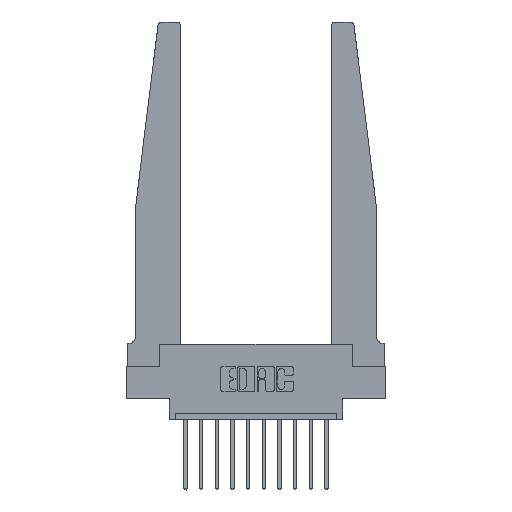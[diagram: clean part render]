
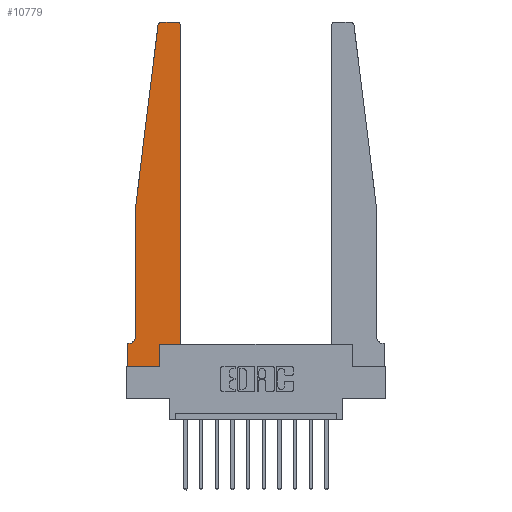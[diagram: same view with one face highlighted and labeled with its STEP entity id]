
A CAD part, top view. The second image highlights one B-rep face of the part: STEP entity #10779.
In plain terms, the highlighted planar face has unit normal (0, 0, 1).
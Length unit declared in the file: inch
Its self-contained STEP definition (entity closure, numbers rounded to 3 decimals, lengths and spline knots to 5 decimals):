
#94 = EDGE_CURVE ( 'NONE', #14381, #6517, #8369, .T. ) ;
#203 = ORIENTED_EDGE ( 'NONE', *, *, #13547, .T. ) ;
#266 = EDGE_CURVE ( 'NONE', #2479, #7509, #4620, .T. ) ;
#385 = DIRECTION ( 'NONE',  ( -1., 0., 0. ) ) ;
#574 = EDGE_CURVE ( 'NONE', #6517, #11387, #15032, .T. ) ;
#618 = CARTESIAN_POINT ( 'NONE',  ( 0.24675, 2.72367, 0.37 ) ) ;
#689 = EDGE_CURVE ( 'NONE', #11387, #13589, #2000, .T. ) ;
#945 = CARTESIAN_POINT ( 'NONE',  ( 0., 0., 0.37 ) ) ;
#994 = LINE ( 'NONE', #6696, #12910 ) ;
#1380 = DIRECTION ( 'NONE',  ( 0., 1., 0. ) ) ;
#1482 = VECTOR ( 'NONE', #5761, 39.37008 ) ;
#1669 = LINE ( 'NONE', #9377, #1482 ) ;
#1726 = CARTESIAN_POINT ( 'NONE',  ( 0., 0.1875, 0.37 ) ) ;
#1998 = ORIENTED_EDGE ( 'NONE', *, *, #94, .T. ) ;
#2000 = CIRCLE ( 'NONE', #4517, 0.05 ) ;
#2479 = VERTEX_POINT ( 'NONE', #14240 ) ;
#2509 = DIRECTION ( 'NONE',  ( 1., 0., 0. ) ) ;
#2697 = CARTESIAN_POINT ( 'NONE',  ( 0., 0.1875, 0.37 ) ) ;
#2718 = LINE ( 'NONE', #7629, #4381 ) ;
#2761 = EDGE_CURVE ( 'NONE', #13950, #14381, #3638, .T. ) ;
#2949 = ORIENTED_EDGE ( 'NONE', *, *, #2761, .T. ) ;
#3106 = ORIENTED_EDGE ( 'NONE', *, *, #574, .T. ) ;
#3379 = CARTESIAN_POINT ( 'NONE',  ( 0.2605, 0.18, 0.37 ) ) ;
#3638 = CIRCLE ( 'NONE', #13577, 0.03 ) ;
#3648 = CARTESIAN_POINT ( 'NONE',  ( 0.395, 2.75, 0.37 ) ) ;
#3850 = CARTESIAN_POINT ( 'NONE',  ( 0.27653, 2.72, 0.37 ) ) ;
#3911 = DIRECTION ( 'NONE',  ( 1., 0., 0. ) ) ;
#4058 = ORIENTED_EDGE ( 'NONE', *, *, #11117, .T. ) ;
#4083 = LINE ( 'NONE', #11923, #5564 ) ;
#4130 = CARTESIAN_POINT ( 'NONE',  ( 0.25, 2.75, 0.37 ) ) ;
#4381 = VECTOR ( 'NONE', #7582, 39.37008 ) ;
#4398 = CARTESIAN_POINT ( 'NONE',  ( 0.27653, 2.75, 0.37 ) ) ;
#4490 = CIRCLE ( 'NONE', #13267, 0.03 ) ;
#4517 = AXIS2_PLACEMENT_3D ( 'NONE', #7605, #12346, #385 ) ;
#4620 = LINE ( 'NONE', #8796, #14852 ) ;
#5473 = CARTESIAN_POINT ( 'NONE',  ( 0.065, 0.2375, 0.37 ) ) ;
#5564 = VECTOR ( 'NONE', #1380, 39.37008 ) ;
#5761 = DIRECTION ( 'NONE',  ( 0., -1., 0. ) ) ;
#5963 = CARTESIAN_POINT ( 'NONE',  ( 0.065, 1.25, 0.37 ) ) ;
#6069 = CARTESIAN_POINT ( 'NONE',  ( 0.065, 1.25, 0.37 ) ) ;
#6158 = ORIENTED_EDGE ( 'NONE', *, *, #15377, .T. ) ;
#6278 = VECTOR ( 'NONE', #8907, 39.37008 ) ;
#6314 = CARTESIAN_POINT ( 'NONE',  ( 0.015, 0.1875, 0.37 ) ) ;
#6318 = CARTESIAN_POINT ( 'NONE',  ( 0.065, 1.25, 0.37 ) ) ;
#6517 = VERTEX_POINT ( 'NONE', #5963 ) ;
#6696 = CARTESIAN_POINT ( 'NONE',  ( 0., 0., 0.37 ) ) ;
#7171 = CARTESIAN_POINT ( 'NONE',  ( 0.395, 2.72, 0.37 ) ) ;
#7348 = ORIENTED_EDGE ( 'NONE', *, *, #10474, .T. ) ;
#7509 = VERTEX_POINT ( 'NONE', #3379 ) ;
#7582 = DIRECTION ( 'NONE',  ( -1., 0., 0. ) ) ;
#7605 = CARTESIAN_POINT ( 'NONE',  ( 0.015, 0.2375, 0.37 ) ) ;
#7629 = CARTESIAN_POINT ( 'NONE',  ( 0.065, 0.1875, 0.37 ) ) ;
#7836 = VERTEX_POINT ( 'NONE', #8964 ) ;
#8135 = VECTOR ( 'NONE', #9257, 39.37008 ) ;
#8369 = LINE ( 'NONE', #6069, #10794 ) ;
#8403 = EDGE_CURVE ( 'NONE', #8819, #13950, #13340, .T. ) ;
#8549 = DIRECTION ( 'NONE',  ( 0., 0., 1. ) ) ;
#8582 = AXIS2_PLACEMENT_3D ( 'NONE', #2697, #11016, #3911 ) ;
#8670 = EDGE_CURVE ( 'NONE', #7509, #7836, #12239, .T. ) ;
#8701 = DIRECTION ( 'NONE',  ( 0., 1., 0. ) ) ;
#8796 = CARTESIAN_POINT ( 'NONE',  ( 0.2605, 0.18, 0.37 ) ) ;
#8819 = VERTEX_POINT ( 'NONE', #3648 ) ;
#8888 = ORIENTED_EDGE ( 'NONE', *, *, #8670, .T. ) ;
#8907 = DIRECTION ( 'NONE',  ( -1., 0., 0. ) ) ;
#8964 = CARTESIAN_POINT ( 'NONE',  ( 0.425, 0.18, 0.37 ) ) ;
#9257 = DIRECTION ( 'NONE',  ( 1., 0., 0. ) ) ;
#9377 = CARTESIAN_POINT ( 'NONE',  ( 0., 0., 0.37 ) ) ;
#9619 = EDGE_LOOP ( 'NONE', ( #9907, #2949, #1998, #3106, #12048, #6158, #14866, #7348, #12323, #8888, #203, #4058 ) ) ;
#9646 = DIRECTION ( 'NONE',  ( 0., 0., 1. ) ) ;
#9656 = DIRECTION ( 'NONE',  ( -0.122, -0.992, 0. ) ) ;
#9907 = ORIENTED_EDGE ( 'NONE', *, *, #8403, .T. ) ;
#10283 = VERTEX_POINT ( 'NONE', #11027 ) ;
#10285 = DIRECTION ( 'NONE',  ( 1., 0., 0. ) ) ;
#10474 = EDGE_CURVE ( 'NONE', #15164, #2479, #994, .T. ) ;
#10578 = EDGE_CURVE ( 'NONE', #15374, #15164, #1669, .T. ) ;
#10779 = ADVANCED_FACE ( 'NONE', ( #14742 ), #14711, .T. ) ;
#10794 = VECTOR ( 'NONE', #9656, 39.37008 ) ;
#11016 = DIRECTION ( 'NONE',  ( 0., 0., 1. ) ) ;
#11027 = CARTESIAN_POINT ( 'NONE',  ( 0.425, 2.72, 0.37 ) ) ;
#11117 = EDGE_CURVE ( 'NONE', #10283, #8819, #4490, .T. ) ;
#11387 = VERTEX_POINT ( 'NONE', #5473 ) ;
#11840 = VECTOR ( 'NONE', #14461, 39.37008 ) ;
#11923 = CARTESIAN_POINT ( 'NONE',  ( 0.425, 0.18, 0.37 ) ) ;
#12048 = ORIENTED_EDGE ( 'NONE', *, *, #689, .T. ) ;
#12239 = LINE ( 'NONE', #15186, #8135 ) ;
#12323 = ORIENTED_EDGE ( 'NONE', *, *, #266, .T. ) ;
#12346 = DIRECTION ( 'NONE',  ( 0., 0., -1. ) ) ;
#12910 = VECTOR ( 'NONE', #10285, 39.37008 ) ;
#13267 = AXIS2_PLACEMENT_3D ( 'NONE', #7171, #9646, #2509 ) ;
#13340 = LINE ( 'NONE', #4130, #6278 ) ;
#13547 = EDGE_CURVE ( 'NONE', #7836, #10283, #4083, .T. ) ;
#13577 = AXIS2_PLACEMENT_3D ( 'NONE', #3850, #8549, #14606 ) ;
#13589 = VERTEX_POINT ( 'NONE', #6314 ) ;
#13950 = VERTEX_POINT ( 'NONE', #4398 ) ;
#14240 = CARTESIAN_POINT ( 'NONE',  ( 0.2605, 0., 0.37 ) ) ;
#14381 = VERTEX_POINT ( 'NONE', #618 ) ;
#14461 = DIRECTION ( 'NONE',  ( 0., -1., 0. ) ) ;
#14606 = DIRECTION ( 'NONE',  ( 1., 0., 0. ) ) ;
#14711 = PLANE ( 'NONE',  #8582 ) ;
#14742 = FACE_OUTER_BOUND ( 'NONE', #9619, .T. ) ;
#14852 = VECTOR ( 'NONE', #8701, 39.37008 ) ;
#14866 = ORIENTED_EDGE ( 'NONE', *, *, #10578, .T. ) ;
#15032 = LINE ( 'NONE', #6318, #11840 ) ;
#15164 = VERTEX_POINT ( 'NONE', #945 ) ;
#15186 = CARTESIAN_POINT ( 'NONE',  ( 0.425, 0.18, 0.37 ) ) ;
#15374 = VERTEX_POINT ( 'NONE', #1726 ) ;
#15377 = EDGE_CURVE ( 'NONE', #13589, #15374, #2718, .T. ) ;
